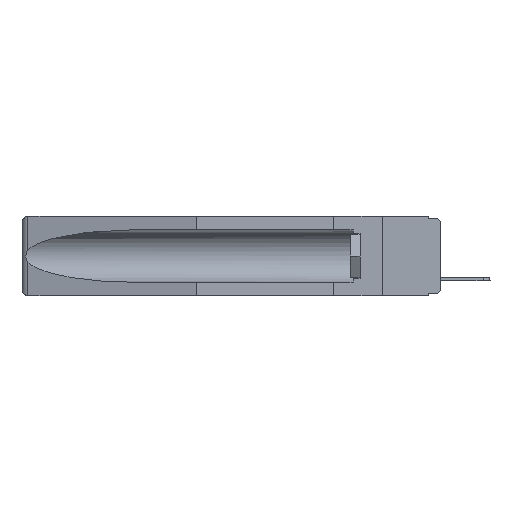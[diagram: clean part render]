
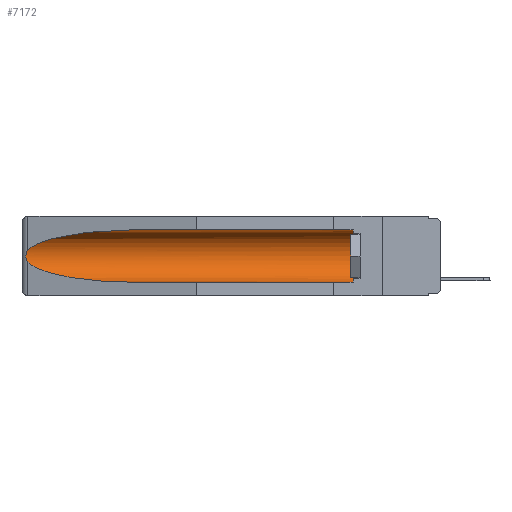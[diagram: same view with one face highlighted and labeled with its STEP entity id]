
A CAD part, left-side view. The second image highlights one B-rep face of the part: STEP entity #7172.
In plain terms, the highlighted cylindrical face has radius 2.857 mm (diameter 5.715 mm), a partial arc.
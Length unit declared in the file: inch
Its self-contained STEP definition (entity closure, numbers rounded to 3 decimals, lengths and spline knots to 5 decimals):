
#240 = DIRECTION ( 'NONE',  ( 0., 0., 1. ) ) ;
#554 = VERTEX_POINT ( 'NONE', #6371 ) ;
#760 = DIRECTION ( 'NONE',  ( 0., 1., 0. ) ) ;
#1665 = VERTEX_POINT ( 'NONE', #17031 ) ;
#1693 = ORIENTED_EDGE ( 'NONE', *, *, #20101, .T. ) ;
#2014 = VERTEX_POINT ( 'NONE', #13480 ) ;
#2276 = VERTEX_POINT ( 'NONE', #9255 ) ;
#2289 = CIRCLE ( 'NONE', #13898, 0.1125 ) ;
#3209 = CYLINDRICAL_SURFACE ( 'NONE', #12060, 0.1125 ) ;
#3249 = CARTESIAN_POINT ( 'NONE',  ( 0.155, 0.126, -0.284 ) ) ;
#3943 = CARTESIAN_POINT ( 'NONE',  ( 0.25451, 1.48313, -0.09465 ) ) ;
#4852 = CARTESIAN_POINT ( 'NONE',  ( 0.2673, 1.5327, -0.16383 ) ) ;
#6272 = LINE ( 'NONE', #22269, #11980 ) ;
#6371 = CARTESIAN_POINT ( 'NONE',  ( 0.155, 1.07973, -0.284 ) ) ;
#6540 = ORIENTED_EDGE ( 'NONE', *, *, #11853, .F. ) ;
#6606 = CARTESIAN_POINT ( 'NONE',  ( 0.2675, 1.53308, -0.17534 ) ) ;
#6702 = CARTESIAN_POINT ( 'NONE',  ( 0.21114, 1.30732, -0.284 ) ) ;
#6854 = CARTESIAN_POINT ( 'NONE',  ( 0.26537, 1.52718, -0.14972 ) ) ;
#7014 = B_SPLINE_CURVE_WITH_KNOTS ( 'NONE', 3,
 ( #6854, #15617, #22602, #4852, #15396, #6606, #19233, #17370, #22839, #13994 ),
 .UNSPECIFIED., .F., .F.,
 ( 4, 2, 2, 2, 4 ),
 ( 0., 0.00029, 0.00058, 0.00087, 0.00117 ),
 .UNSPECIFIED. ) ;
#7051 = DIRECTION ( 'NONE',  ( 0., -1., 0. ) ) ;
#7172 = ADVANCED_FACE ( 'NONE', ( #19122 ), #3209, .F. ) ;
#7302 = CARTESIAN_POINT ( 'NONE',  ( 0.155, 0.126, -0.1715 ) ) ;
#7465 = CARTESIAN_POINT ( 'NONE',  ( 0.26537, 1.52718, -0.14972 ) ) ;
#8127 = CARTESIAN_POINT ( 'NONE',  ( 0.155, 1.07973, -0.284 ) ) ;
#8382 = DIRECTION ( 'NONE',  ( 0., 0., 1. ) ) ;
#8580 = CARTESIAN_POINT ( 'NONE',  ( 0.26537, 1.52718, -0.19328 ) ) ;
#9113 = EDGE_CURVE ( 'NONE', #2014, #2276, #6272, .T. ) ;
#9255 = CARTESIAN_POINT ( 'NONE',  ( 0.155, 1.07973, -0.059 ) ) ;
#10127 = ORIENTED_EDGE ( 'NONE', *, *, #19316, .T. ) ;
#11013 = EDGE_CURVE ( 'NONE', #1665, #554, #15917, .T. ) ;
#11670 = DIRECTION ( 'NONE',  ( 0., 1., 0. ) ) ;
#11853 = EDGE_CURVE ( 'NONE', #16603, #554, #13661, .T. ) ;
#11980 = VECTOR ( 'NONE', #760, 39.37008 ) ;
#12060 = AXIS2_PLACEMENT_3D ( 'NONE', #17480, #11670, #8382 ) ;
#12642 = ORIENTED_EDGE ( 'NONE', *, *, #11013, .T. ) ;
#12855 = CARTESIAN_POINT ( 'NONE',  ( 0.21114, 1.30732, -0.059 ) ) ;
#13480 = CARTESIAN_POINT ( 'NONE',  ( 0.155, 0.126, -0.059 ) ) ;
#13661 = LINE ( 'NONE', #20765, #19478 ) ;
#13898 = AXIS2_PLACEMENT_3D ( 'NONE', #7302, #7051, #240 ) ;
#13994 = CARTESIAN_POINT ( 'NONE',  ( 0.26537, 1.52718, -0.19328 ) ) ;
#14378 = CARTESIAN_POINT ( 'NONE',  ( 0.155, 1.07973, -0.059 ) ) ;
#15396 = CARTESIAN_POINT ( 'NONE',  ( 0.2675, 1.53308, -0.16763 ) ) ;
#15617 = CARTESIAN_POINT ( 'NONE',  ( 0.26597, 1.52961, -0.15275 ) ) ;
#15769 =( BOUNDED_CURVE ( )  B_SPLINE_CURVE ( 3, ( #14378, #12855, #3943, #21475 ),
 .UNSPECIFIED., .F., .F. ) 
 B_SPLINE_CURVE_WITH_KNOTS ( ( 4, 4 ),
 ( 4.71239, 6.08839 ),
 .UNSPECIFIED. ) 
 CURVE ( )  GEOMETRIC_REPRESENTATION_ITEM ( )  RATIONAL_B_SPLINE_CURVE ( ( 1., 0.848, 0.848, 1. ) ) 
 REPRESENTATION_ITEM ( '' )  );
#15917 =( BOUNDED_CURVE ( )  B_SPLINE_CURVE ( 3, ( #8580, #22816, #6702, #8127 ),
 .UNSPECIFIED., .F., .F. ) 
 B_SPLINE_CURVE_WITH_KNOTS ( ( 4, 4 ),
 ( 0.1948, 1.5708 ),
 .UNSPECIFIED. ) 
 CURVE ( )  GEOMETRIC_REPRESENTATION_ITEM ( )  RATIONAL_B_SPLINE_CURVE ( ( 1., 0.848, 0.848, 1. ) ) 
 REPRESENTATION_ITEM ( '' )  );
#16478 = ORIENTED_EDGE ( 'NONE', *, *, #20824, .T. ) ;
#16603 = VERTEX_POINT ( 'NONE', #3249 ) ;
#17031 = CARTESIAN_POINT ( 'NONE',  ( 0.26537, 1.52718, -0.19328 ) ) ;
#17370 = CARTESIAN_POINT ( 'NONE',  ( 0.26655, 1.53094, -0.18657 ) ) ;
#17480 = CARTESIAN_POINT ( 'NONE',  ( 0.155, -0.30754, -0.1715 ) ) ;
#19122 = FACE_OUTER_BOUND ( 'NONE', #21496, .T. ) ;
#19233 = CARTESIAN_POINT ( 'NONE',  ( 0.2673, 1.53269, -0.17917 ) ) ;
#19303 = VERTEX_POINT ( 'NONE', #7465 ) ;
#19316 = EDGE_CURVE ( 'NONE', #2276, #19303, #15769, .T. ) ;
#19478 = VECTOR ( 'NONE', #21217, 39.37008 ) ;
#20101 = EDGE_CURVE ( 'NONE', #16603, #2014, #2289, .T. ) ;
#20765 = CARTESIAN_POINT ( 'NONE',  ( 0.155, -0.30754, -0.284 ) ) ;
#20824 = EDGE_CURVE ( 'NONE', #19303, #1665, #7014, .T. ) ;
#21217 = DIRECTION ( 'NONE',  ( 0., 1., 0. ) ) ;
#21475 = CARTESIAN_POINT ( 'NONE',  ( 0.26537, 1.52718, -0.14972 ) ) ;
#21496 = EDGE_LOOP ( 'NONE', ( #10127, #16478, #12642, #6540, #1693, #22549 ) ) ;
#22269 = CARTESIAN_POINT ( 'NONE',  ( 0.155, -0.30754, -0.059 ) ) ;
#22549 = ORIENTED_EDGE ( 'NONE', *, *, #9113, .T. ) ;
#22602 = CARTESIAN_POINT ( 'NONE',  ( 0.26654, 1.53092, -0.15636 ) ) ;
#22816 = CARTESIAN_POINT ( 'NONE',  ( 0.25451, 1.48313, -0.24835 ) ) ;
#22839 = CARTESIAN_POINT ( 'NONE',  ( 0.26597, 1.5296, -0.19026 ) ) ;
